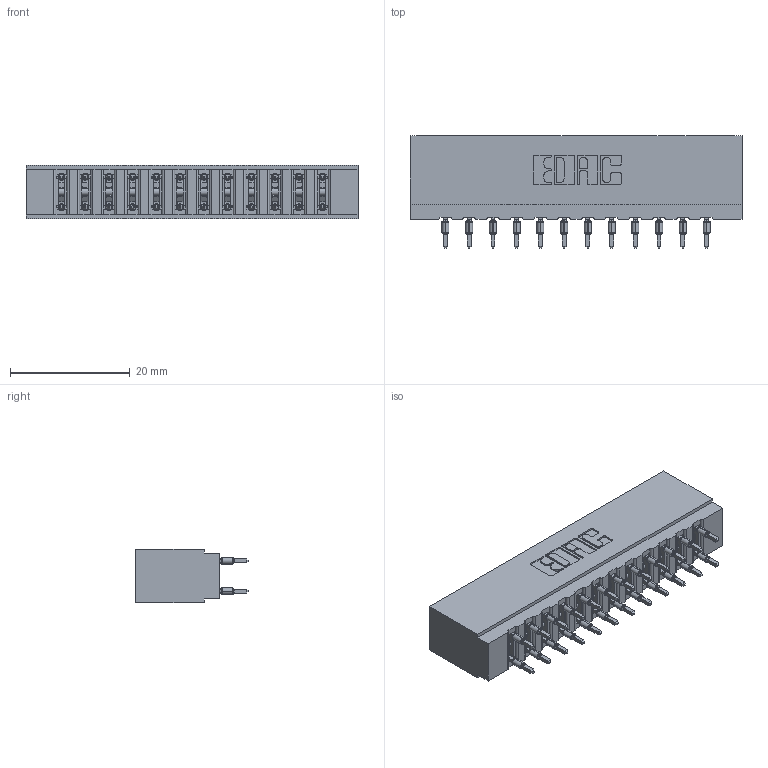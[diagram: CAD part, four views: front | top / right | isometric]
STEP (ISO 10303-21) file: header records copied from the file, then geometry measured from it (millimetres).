
FILE_DESCRIPTION (( 'STEP AP203' ), '1' );
FILE_NAME ('717-024-560-201.STEP', '2026-02-20T17:23:00', ( '' ), ( '' ), 'SwSTEP 2.0', 'SolidWorks 2023', '' );
FILE_SCHEMA (( 'CONFIG_CONTROL_DESIGN' ));
Length unit declared in the file: millimetre
Products named in the file (3): 717-024-560-201; 717 Part_Insulator Option - 06; 745-292-001_560
Assembly tree (25 placements, depth 2):
  717-024-560-201
    717 Part_Insulator Option - 06
    745-292-001_560  x24
Bounding box: 55.42 x 18.78 x 8.89 mm (x, y, z)
Volume: 5015.1 mm3; surface area: 7691.2 mm2
Topology: 25 solids, 25 shells, 2470 faces, 6755 edges, 4294 vertices
Faces by surface type: plane 1290, cylinder 556, bspline 480, torus 144
Entity records: 24948 total; most frequent: CARTESIAN_POINT 4843, ORIENTED_EDGE 4218, DIRECTION 3715, EDGE_CURVE 2109, VECTOR 1847, LINE 1847, VERTEX_POINT 1350, AXIS2_PLACEMENT_3D 934
